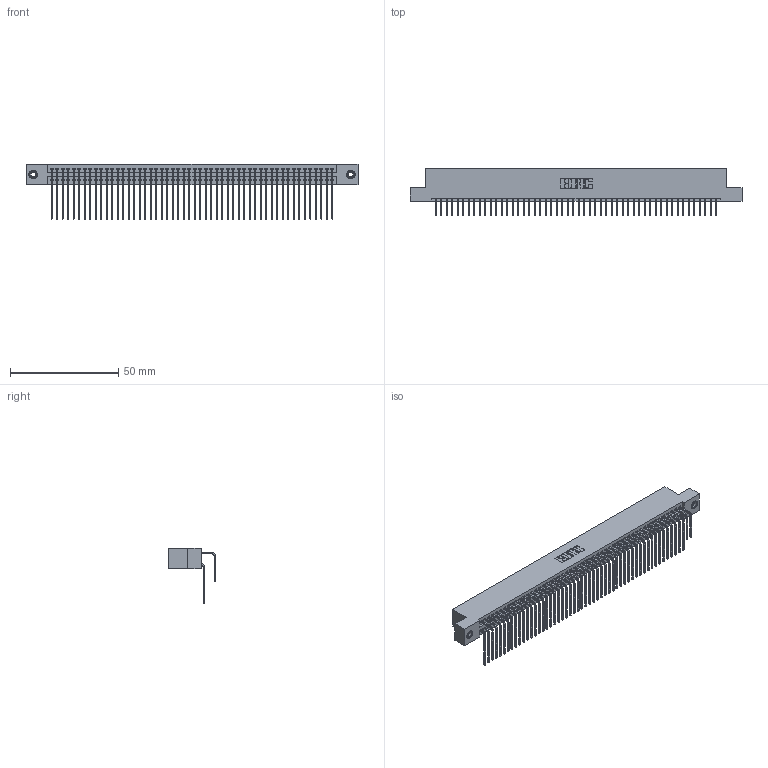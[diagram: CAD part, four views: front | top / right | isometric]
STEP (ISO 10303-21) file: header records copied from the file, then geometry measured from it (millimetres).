
FILE_DESCRIPTION (( 'STEP AP203' ), '1' );
FILE_NAME ('345-104-558-208.STEP', '2018-10-06T01:26:49', ( '' ), ( '' ), 'SwSTEP 2.0', 'SolidWorks 2016', '' );
FILE_SCHEMA (( 'CONFIG_CONTROL_DESIGN' ));
Length unit declared in the file: inch
Products named in the file (5): 345-292-001_558 559 Tail - 1; 345 Part_Flush Mounting Lugs - 0.156 Dia-TI; 345-250-001_345-250-003-102; 345-292-001_558 Tail - 2; 345-104-558-208
Assembly tree (107 placements, depth 2):
  345-104-558-208
    345 Part_Flush Mounting Lugs - 0.156 Dia-TI
    345-292-001_558 559 Tail - 1  x52
    345-292-001_558 Tail - 2  x52
    345-250-001_345-250-003-102  x2
Bounding box: 153.29 x 21.83 x 25.53 mm (x, y, z)
Volume: 15576.9 mm3; surface area: 26053.5 mm2
Topology: 107 solids, 107 shells, 5594 faces, 16597 edges, 10918 vertices
Faces by surface type: plane 3752, cylinder 1826, cone 12, torus 4
Entity records: 42292 total; most frequent: CARTESIAN_POINT 7106, ORIENTED_EDGE 6982, DIRECTION 6253, EDGE_CURVE 3491, VECTOR 3091, LINE 3091, VERTEX_POINT 2320, AXIS2_PLACEMENT_3D 1581
